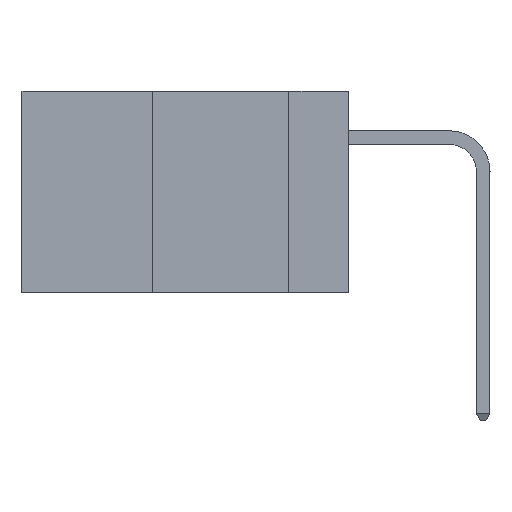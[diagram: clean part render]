
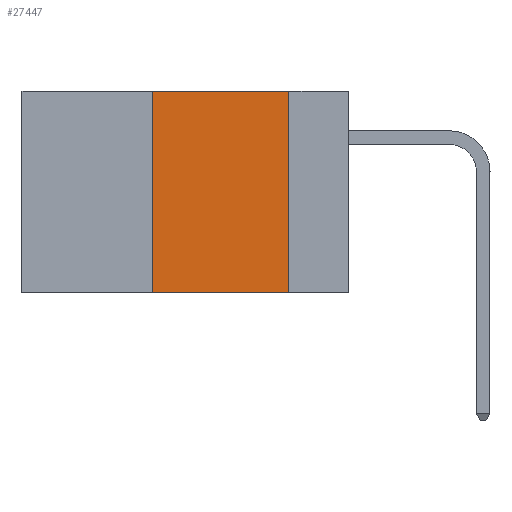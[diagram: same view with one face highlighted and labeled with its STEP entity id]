
A CAD part, left-side view. The second image highlights one B-rep face of the part: STEP entity #27447.
In plain terms, the highlighted planar face has unit normal (-1, 0, 0).
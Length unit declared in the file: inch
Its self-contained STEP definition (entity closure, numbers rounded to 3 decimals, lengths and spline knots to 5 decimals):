
#950 = CARTESIAN_POINT ( 'NONE',  ( 0., 0.11, 0. ) ) ;
#1448 = PLANE ( 'NONE',  #16081 ) ;
#1936 = ORIENTED_EDGE ( 'NONE', *, *, #25911, .F. ) ;
#2160 = ORIENTED_EDGE ( 'NONE', *, *, #15991, .F. ) ;
#3128 = DIRECTION ( 'NONE',  ( 0., 0., 1. ) ) ;
#3157 = EDGE_LOOP ( 'NONE', ( #1936, #26206, #2160, #27138 ) ) ;
#3696 = VECTOR ( 'NONE', #13748, 39.37008 ) ;
#6732 = LINE ( 'NONE', #25539, #37885 ) ;
#6923 = CARTESIAN_POINT ( 'NONE',  ( 0., 0.6, 0. ) ) ;
#7733 = CARTESIAN_POINT ( 'NONE',  ( 0., 0.36, -0.37 ) ) ;
#8073 = VERTEX_POINT ( 'NONE', #7733 ) ;
#8093 = VECTOR ( 'NONE', #10783, 39.37008 ) ;
#10742 = EDGE_CURVE ( 'NONE', #18847, #16414, #20999, .T. ) ;
#10783 = DIRECTION ( 'NONE',  ( 0., 0., -1. ) ) ;
#11670 = CARTESIAN_POINT ( 'NONE',  ( 0., 0.6, -0.37 ) ) ;
#13015 = FACE_OUTER_BOUND ( 'NONE', #3157, .T. ) ;
#13544 = LINE ( 'NONE', #11670, #39630 ) ;
#13738 = CARTESIAN_POINT ( 'NONE',  ( 0., 0.36, 0. ) ) ;
#13748 = DIRECTION ( 'NONE',  ( 0., -1., 0. ) ) ;
#13956 = CARTESIAN_POINT ( 'NONE',  ( 0., 0.11, 0. ) ) ;
#14946 = DIRECTION ( 'NONE',  ( 0., -1., 0. ) ) ;
#15196 = LINE ( 'NONE', #950, #8093 ) ;
#15991 = EDGE_CURVE ( 'NONE', #8073, #18847, #6732, .T. ) ;
#16081 = AXIS2_PLACEMENT_3D ( 'NONE', #24185, #37220, #40570 ) ;
#16414 = VERTEX_POINT ( 'NONE', #13956 ) ;
#18847 = VERTEX_POINT ( 'NONE', #13738 ) ;
#19448 = VERTEX_POINT ( 'NONE', #23191 ) ;
#20999 = LINE ( 'NONE', #6923, #3696 ) ;
#21075 = EDGE_CURVE ( 'NONE', #8073, #19448, #13544, .T. ) ;
#23191 = CARTESIAN_POINT ( 'NONE',  ( 0., 0.11, -0.37 ) ) ;
#24185 = CARTESIAN_POINT ( 'NONE',  ( 0., 0.6, 0. ) ) ;
#25539 = CARTESIAN_POINT ( 'NONE',  ( 0., 0.36, 0. ) ) ;
#25911 = EDGE_CURVE ( 'NONE', #16414, #19448, #15196, .T. ) ;
#26206 = ORIENTED_EDGE ( 'NONE', *, *, #10742, .F. ) ;
#27138 = ORIENTED_EDGE ( 'NONE', *, *, #21075, .T. ) ;
#27447 = ADVANCED_FACE ( 'NONE', ( #13015 ), #1448, .F. ) ;
#37220 = DIRECTION ( 'NONE',  ( 1., 0., 0. ) ) ;
#37885 = VECTOR ( 'NONE', #3128, 39.37008 ) ;
#39630 = VECTOR ( 'NONE', #14946, 39.37008 ) ;
#40570 = DIRECTION ( 'NONE',  ( 0., 0., -1. ) ) ;
